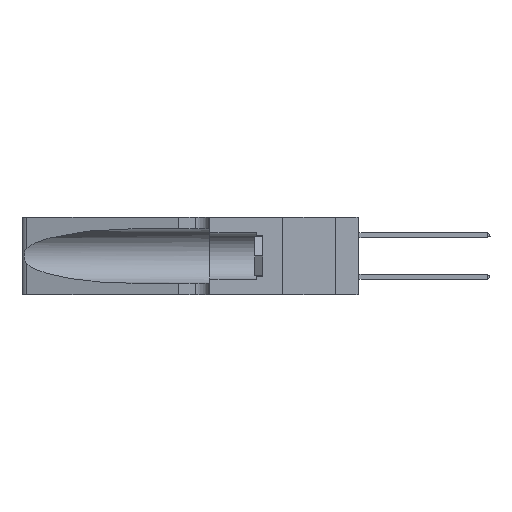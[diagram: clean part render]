
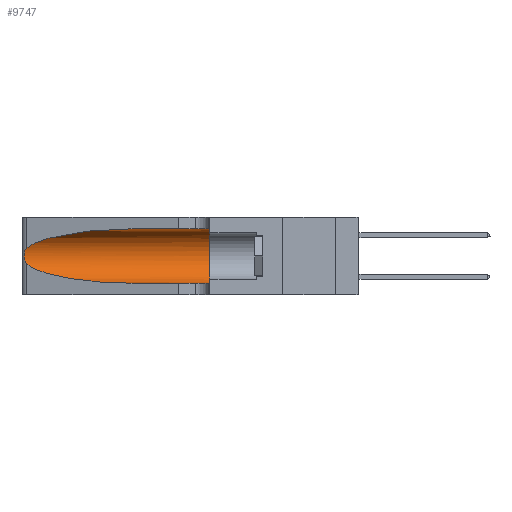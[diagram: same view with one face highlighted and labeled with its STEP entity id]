
A CAD part, left-side view. The second image highlights one B-rep face of the part: STEP entity #9747.
In plain terms, the highlighted cylindrical face has radius 3.308 mm (diameter 6.617 mm), a partial arc.
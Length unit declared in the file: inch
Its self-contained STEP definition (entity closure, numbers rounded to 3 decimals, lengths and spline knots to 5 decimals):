
#634 = VERTEX_POINT ( 'NONE', #23241 ) ;
#770 = DIRECTION ( 'NONE',  ( 0., 0., 1. ) ) ;
#1235 = CARTESIAN_POINT ( 'NONE',  ( 0.25787, 1.23484, 0.2124 ) ) ;
#1475 = VECTOR ( 'NONE', #7905, 39.37008 ) ;
#3189 = CYLINDRICAL_SURFACE ( 'NONE', #43417, 0.13025 ) ;
#3863 = CARTESIAN_POINT ( 'NONE',  ( 0.1305, 0.35, 0.31525 ) ) ;
#4752 = CARTESIAN_POINT ( 'NONE',  ( 0.26018, 1.23835, 0.19895 ) ) ;
#6009 = EDGE_CURVE ( 'NONE', #37877, #41584, #29396, .T. ) ;
#7233 = VERTEX_POINT ( 'NONE', #3863 ) ;
#7905 = DIRECTION ( 'NONE',  ( 0., -1., 0. ) ) ;
#8125 = CARTESIAN_POINT ( 'NONE',  ( 0.25555, 1.22994, 0.2215 ) ) ;
#8280 = CARTESIAN_POINT ( 'NONE',  ( 0.26075, 1.23896, 0.178 ) ) ;
#9392 = CARTESIAN_POINT ( 'NONE',  ( 0.1305, 1.61858, 0.185 ) ) ;
#9544 = DIRECTION ( 'NONE',  ( 0., -1., 0. ) ) ;
#9747 = ADVANCED_FACE ( 'NONE', ( #43387 ), #3189, .F. ) ;
#10323 = CARTESIAN_POINT ( 'NONE',  ( 0.25487, 1.22718, 0.14631 ) ) ;
#11188 = CARTESIAN_POINT ( 'NONE',  ( 0.25487, 1.22718, 0.22369 ) ) ;
#11464 = CARTESIAN_POINT ( 'NONE',  ( 0.1305, 1.61858, 0.05475 ) ) ;
#11845 = CARTESIAN_POINT ( 'NONE',  ( 0.25856, 1.23593, 0.16098 ) ) ;
#12420 = ORIENTED_EDGE ( 'NONE', *, *, #14022, .T. ) ;
#12538 = CIRCLE ( 'NONE', #44587, 0.13025 ) ;
#12622 = ORIENTED_EDGE ( 'NONE', *, *, #19285, .T. ) ;
#14022 = EDGE_CURVE ( 'NONE', #25947, #14095, #21579, .T. ) ;
#14095 = VERTEX_POINT ( 'NONE', #26219 ) ;
#15263 = CARTESIAN_POINT ( 'NONE',  ( 0.25639, 1.23184, 0.21858 ) ) ;
#15410 = CARTESIAN_POINT ( 'NONE',  ( 0.25639, 1.23186, 0.15144 ) ) ;
#15487 = EDGE_CURVE ( 'NONE', #634, #7233, #22236, .T. ) ;
#15498 = ORIENTED_EDGE ( 'NONE', *, *, #6009, .T. ) ;
#17416 = CARTESIAN_POINT ( 'NONE',  ( 0.18966, 0.96281, 0.05475 ) ) ;
#18932 = CARTESIAN_POINT ( 'NONE',  ( 0.25487, 1.22718, 0.14631 ) ) ;
#19285 = EDGE_CURVE ( 'NONE', #14095, #37877, #42256, .T. ) ;
#20088 = CARTESIAN_POINT ( 'NONE',  ( 0.2373, 1.15595, 0.28018 ) ) ;
#21007 = EDGE_CURVE ( 'NONE', #634, #25947, #34312, .T. ) ;
#21579 = B_SPLINE_CURVE_WITH_KNOTS ( 'NONE', 3,
 ( #42841, #8125, #15263, #1235, #25749, #4752, #29225, #8280, #32662, #11845, #36108, #15410, #39563, #18932 ),
 .UNSPECIFIED., .F., .F.,
 ( 4, 2, 2, 2, 2, 2, 4 ),
 ( 0., 0.00027, 0.00053, 0.00107, 0.0016, 0.00187, 0.00214 ),
 .UNSPECIFIED. ) ;
#21801 = DIRECTION ( 'NONE',  ( 0., 1., 0. ) ) ;
#22236 = LINE ( 'NONE', #33631, #40546 ) ;
#23241 = CARTESIAN_POINT ( 'NONE',  ( 0.1305, 0.72297, 0.31525 ) ) ;
#25749 = CARTESIAN_POINT ( 'NONE',  ( 0.25854, 1.2359, 0.20912 ) ) ;
#25947 = VERTEX_POINT ( 'NONE', #11188 ) ;
#26219 = CARTESIAN_POINT ( 'NONE',  ( 0.25487, 1.22718, 0.14631 ) ) ;
#26272 = CARTESIAN_POINT ( 'NONE',  ( 0.1305, 0.35, 0.05475 ) ) ;
#26817 = CARTESIAN_POINT ( 'NONE',  ( 0.1305, 0.72297, 0.05475 ) ) ;
#26977 = DIRECTION ( 'NONE',  ( 0., 0., -1. ) ) ;
#29225 = CARTESIAN_POINT ( 'NONE',  ( 0.26075, 1.23896, 0.19203 ) ) ;
#29396 = LINE ( 'NONE', #11464, #1475 ) ;
#31201 = CARTESIAN_POINT ( 'NONE',  ( 0.2373, 1.15595, 0.08982 ) ) ;
#31435 = EDGE_CURVE ( 'NONE', #7233, #41584, #12538, .T. ) ;
#32662 = CARTESIAN_POINT ( 'NONE',  ( 0.26017, 1.23833, 0.17102 ) ) ;
#33631 = CARTESIAN_POINT ( 'NONE',  ( 0.1305, 1.61858, 0.31525 ) ) ;
#34312 =( BOUNDED_CURVE ( )  B_SPLINE_CURVE ( 3, ( #37246, #40700, #20088, #44162 ),
 .UNSPECIFIED., .F., .T. ) 
 B_SPLINE_CURVE_WITH_KNOTS ( ( 4, 4 ),
 ( 1.5708, 2.84003 ),
 .UNSPECIFIED. ) 
 CURVE ( )  GEOMETRIC_REPRESENTATION_ITEM ( )  RATIONAL_B_SPLINE_CURVE ( ( 1., 0.87, 0.87, 1. ) ) 
 REPRESENTATION_ITEM ( '' )  );
#36108 = CARTESIAN_POINT ( 'NONE',  ( 0.25789, 1.23486, 0.15765 ) ) ;
#36581 = EDGE_LOOP ( 'NONE', ( #40408, #12420, #12622, #15498, #40633, #38774 ) ) ;
#37246 = CARTESIAN_POINT ( 'NONE',  ( 0.1305, 0.72297, 0.31525 ) ) ;
#37877 = VERTEX_POINT ( 'NONE', #26817 ) ;
#38774 = ORIENTED_EDGE ( 'NONE', *, *, #15487, .F. ) ;
#39563 = CARTESIAN_POINT ( 'NONE',  ( 0.25555, 1.22993, 0.14849 ) ) ;
#40408 = ORIENTED_EDGE ( 'NONE', *, *, #21007, .T. ) ;
#40546 = VECTOR ( 'NONE', #43824, 39.37008 ) ;
#40633 = ORIENTED_EDGE ( 'NONE', *, *, #31435, .F. ) ;
#40700 = CARTESIAN_POINT ( 'NONE',  ( 0.18966, 0.96281, 0.31525 ) ) ;
#41529 = CARTESIAN_POINT ( 'NONE',  ( 0.1305, 0.72297, 0.05475 ) ) ;
#41584 = VERTEX_POINT ( 'NONE', #26272 ) ;
#42256 =( BOUNDED_CURVE ( )  B_SPLINE_CURVE ( 3, ( #10323, #31201, #17416, #41529 ),
 .UNSPECIFIED., .F., .F. ) 
 B_SPLINE_CURVE_WITH_KNOTS ( ( 4, 4 ),
 ( 3.44316, 4.71239 ),
 .UNSPECIFIED. ) 
 CURVE ( )  GEOMETRIC_REPRESENTATION_ITEM ( )  RATIONAL_B_SPLINE_CURVE ( ( 1., 0.87, 0.87, 1. ) ) 
 REPRESENTATION_ITEM ( '' )  );
#42403 = CARTESIAN_POINT ( 'NONE',  ( 0.1305, 0.35, 0.185 ) ) ;
#42841 = CARTESIAN_POINT ( 'NONE',  ( 0.25487, 1.22718, 0.22369 ) ) ;
#43387 = FACE_OUTER_BOUND ( 'NONE', #36581, .T. ) ;
#43417 = AXIS2_PLACEMENT_3D ( 'NONE', #9392, #9544, #26977 ) ;
#43824 = DIRECTION ( 'NONE',  ( 0., -1., 0. ) ) ;
#44162 = CARTESIAN_POINT ( 'NONE',  ( 0.25487, 1.22718, 0.22369 ) ) ;
#44587 = AXIS2_PLACEMENT_3D ( 'NONE', #42403, #21801, #770 ) ;
